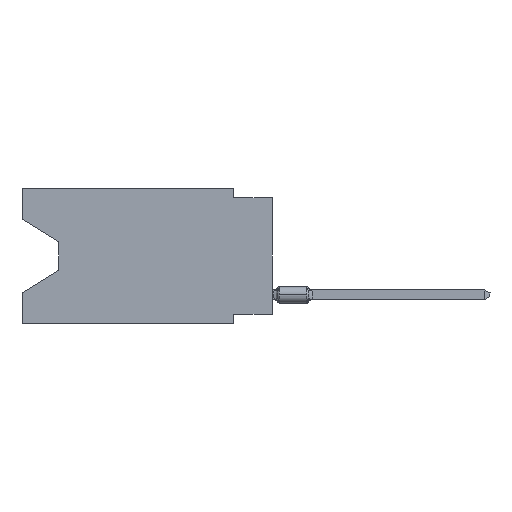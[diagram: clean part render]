
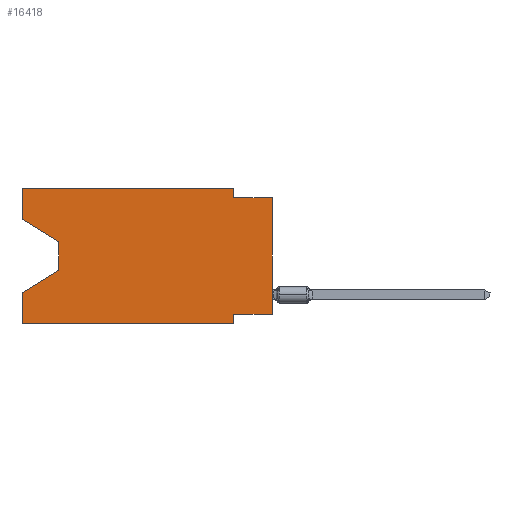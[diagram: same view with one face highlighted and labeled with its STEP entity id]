
A CAD part, left-side view. The second image highlights one B-rep face of the part: STEP entity #16418.
In plain terms, the highlighted planar face has unit normal (-1, 0, 0).
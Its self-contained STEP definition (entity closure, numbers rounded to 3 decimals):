
#2 = LINE ( 'NONE', #21927, #46086 ) ;
#419 = ORIENTED_EDGE ( 'NONE', *, *, #3825, .F. ) ;
#1229 = VERTEX_POINT ( 'NONE', #23318 ) ;
#1656 = EDGE_CURVE ( 'NONE', #2385, #42444, #24972, .T. ) ;
#2029 = DIRECTION ( 'NONE',  ( 0., -1., 0. ) ) ;
#2385 = VERTEX_POINT ( 'NONE', #20226 ) ;
#3034 = CARTESIAN_POINT ( 'NONE',  ( 0., 2.54, -0.635 ) ) ;
#3571 = FACE_OUTER_BOUND ( 'NONE', #19895, .T. ) ;
#3825 = EDGE_CURVE ( 'NONE', #16563, #17031, #41467, .T. ) ;
#4447 = CARTESIAN_POINT ( 'NONE',  ( 0., 16.383, -8.89 ) ) ;
#4960 = EDGE_CURVE ( 'NONE', #27986, #5207, #32942, .T. ) ;
#5034 = DIRECTION ( 'NONE',  ( 0., 0., -1. ) ) ;
#5039 = ORIENTED_EDGE ( 'NONE', *, *, #4960, .T. ) ;
#5207 = VERTEX_POINT ( 'NONE', #31903 ) ;
#5421 = EDGE_CURVE ( 'NONE', #34486, #16563, #33368, .T. ) ;
#6289 = CARTESIAN_POINT ( 'NONE',  ( 0., 2.54, 0. ) ) ;
#6742 = ORIENTED_EDGE ( 'NONE', *, *, #1656, .T. ) ;
#8079 = ORIENTED_EDGE ( 'NONE', *, *, #27293, .F. ) ;
#8285 = AXIS2_PLACEMENT_3D ( 'NONE', #18919, #30460, #45799 ) ;
#8574 = ORIENTED_EDGE ( 'NONE', *, *, #30937, .F. ) ;
#9012 = LINE ( 'NONE', #24568, #41256 ) ;
#9059 = VECTOR ( 'NONE', #11866, 1000. ) ;
#9601 = LINE ( 'NONE', #48049, #35440 ) ;
#9666 = DIRECTION ( 'NONE',  ( 0., -0.855, -0.519 ) ) ;
#10610 = DIRECTION ( 'NONE',  ( 0., 0., 1. ) ) ;
#10812 = DIRECTION ( 'NONE',  ( 0., 0., -1. ) ) ;
#11359 = LINE ( 'NONE', #34215, #9059 ) ;
#11866 = DIRECTION ( 'NONE',  ( 0., -1., 0. ) ) ;
#13371 = DIRECTION ( 'NONE',  ( 0., 0., 1. ) ) ;
#13841 = DIRECTION ( 'NONE',  ( 0., 0.855, -0.519 ) ) ;
#14010 = VECTOR ( 'NONE', #18046, 1000. ) ;
#14646 = VECTOR ( 'NONE', #5034, 1000. ) ;
#16297 = ORIENTED_EDGE ( 'NONE', *, *, #33588, .T. ) ;
#16418 = ADVANCED_FACE ( 'NONE', ( #3571 ), #38516, .F. ) ;
#16563 = VERTEX_POINT ( 'NONE', #47769 ) ;
#16640 = LINE ( 'NONE', #20636, #32888 ) ;
#16718 = CARTESIAN_POINT ( 'NONE',  ( 0., 0., -8.255 ) ) ;
#16900 = ORIENTED_EDGE ( 'NONE', *, *, #31813, .F. ) ;
#17031 = VERTEX_POINT ( 'NONE', #22737 ) ;
#17800 = CARTESIAN_POINT ( 'NONE',  ( 0., 13.97, -3.505 ) ) ;
#18046 = DIRECTION ( 'NONE',  ( 0., 0., -1. ) ) ;
#18372 = CARTESIAN_POINT ( 'NONE',  ( 0., 2.54, -8.89 ) ) ;
#18919 = CARTESIAN_POINT ( 'NONE',  ( 0., 16.383, 0. ) ) ;
#19345 = ORIENTED_EDGE ( 'NONE', *, *, #33767, .T. ) ;
#19820 = VERTEX_POINT ( 'NONE', #6289 ) ;
#19895 = EDGE_LOOP ( 'NONE', ( #6742, #19345, #5039, #42087, #16297, #419, #42692, #38573, #16900, #28901, #8079, #8574 ) ) ;
#20226 = CARTESIAN_POINT ( 'NONE',  ( 0., 16.383, -2.038 ) ) ;
#20636 = CARTESIAN_POINT ( 'NONE',  ( 0., 16.383, 0. ) ) ;
#21433 = VECTOR ( 'NONE', #26128, 1000. ) ;
#21927 = CARTESIAN_POINT ( 'NONE',  ( 0., 0., 0. ) ) ;
#22737 = CARTESIAN_POINT ( 'NONE',  ( 0., 2.54, -8.89 ) ) ;
#23318 = CARTESIAN_POINT ( 'NONE',  ( 0., 16.383, 0. ) ) ;
#24405 = CARTESIAN_POINT ( 'NONE',  ( 0., 0., -0.635 ) ) ;
#24568 = CARTESIAN_POINT ( 'NONE',  ( 0., 16.383, -8.89 ) ) ;
#24972 = LINE ( 'NONE', #28251, #33145 ) ;
#25901 = EDGE_CURVE ( 'NONE', #27479, #5207, #37201, .T. ) ;
#26128 = DIRECTION ( 'NONE',  ( 0., 0., 1. ) ) ;
#26996 = CARTESIAN_POINT ( 'NONE',  ( 0., 13.97, -5.385 ) ) ;
#27293 = EDGE_CURVE ( 'NONE', #1229, #19820, #16640, .T. ) ;
#27479 = VERTEX_POINT ( 'NONE', #4447 ) ;
#27986 = VERTEX_POINT ( 'NONE', #26996 ) ;
#28251 = CARTESIAN_POINT ( 'NONE',  ( 0., 16.383, -2.038 ) ) ;
#28901 = ORIENTED_EDGE ( 'NONE', *, *, #32006, .F. ) ;
#29904 = CARTESIAN_POINT ( 'NONE',  ( 0., 16.383, 0. ) ) ;
#30289 = VECTOR ( 'NONE', #32386, 1000. ) ;
#30460 = DIRECTION ( 'NONE',  ( 1., 0., 0. ) ) ;
#30937 = EDGE_CURVE ( 'NONE', #2385, #1229, #9601, .T. ) ;
#31813 = EDGE_CURVE ( 'NONE', #40453, #38855, #11359, .T. ) ;
#31903 = CARTESIAN_POINT ( 'NONE',  ( 0., 16.383, -6.852 ) ) ;
#32006 = EDGE_CURVE ( 'NONE', #19820, #40453, #43993, .T. ) ;
#32386 = DIRECTION ( 'NONE',  ( 0., 1., 0. ) ) ;
#32888 = VECTOR ( 'NONE', #2029, 1000. ) ;
#32942 = LINE ( 'NONE', #48265, #49487 ) ;
#33145 = VECTOR ( 'NONE', #9666, 1000. ) ;
#33368 = LINE ( 'NONE', #48706, #30289 ) ;
#33432 = EDGE_CURVE ( 'NONE', #34486, #38855, #2, .T. ) ;
#33588 = EDGE_CURVE ( 'NONE', #27479, #17031, #9012, .T. ) ;
#33767 = EDGE_CURVE ( 'NONE', #42444, #27986, #48945, .T. ) ;
#34215 = CARTESIAN_POINT ( 'NONE',  ( 0., 0., -0.635 ) ) ;
#34486 = VERTEX_POINT ( 'NONE', #16718 ) ;
#35440 = VECTOR ( 'NONE', #13371, 1000. ) ;
#36620 = VECTOR ( 'NONE', #10812, 1000. ) ;
#37201 = LINE ( 'NONE', #29904, #21433 ) ;
#38516 = PLANE ( 'NONE',  #8285 ) ;
#38573 = ORIENTED_EDGE ( 'NONE', *, *, #33432, .T. ) ;
#38855 = VERTEX_POINT ( 'NONE', #24405 ) ;
#39479 = CARTESIAN_POINT ( 'NONE',  ( 0., 2.54, 0. ) ) ;
#40168 = DIRECTION ( 'NONE',  ( 0., -1., 0. ) ) ;
#40453 = VERTEX_POINT ( 'NONE', #3034 ) ;
#40880 = CARTESIAN_POINT ( 'NONE',  ( 0., 13.97, -3.505 ) ) ;
#41256 = VECTOR ( 'NONE', #40168, 1000. ) ;
#41467 = LINE ( 'NONE', #18372, #36620 ) ;
#42087 = ORIENTED_EDGE ( 'NONE', *, *, #25901, .F. ) ;
#42444 = VERTEX_POINT ( 'NONE', #40880 ) ;
#42692 = ORIENTED_EDGE ( 'NONE', *, *, #5421, .F. ) ;
#43993 = LINE ( 'NONE', #39479, #14646 ) ;
#45799 = DIRECTION ( 'NONE',  ( 0., 0., -1. ) ) ;
#46086 = VECTOR ( 'NONE', #10610, 1000. ) ;
#47769 = CARTESIAN_POINT ( 'NONE',  ( 0., 2.54, -8.255 ) ) ;
#48049 = CARTESIAN_POINT ( 'NONE',  ( 0., 16.383, 0. ) ) ;
#48265 = CARTESIAN_POINT ( 'NONE',  ( 0., 13.97, -5.385 ) ) ;
#48706 = CARTESIAN_POINT ( 'NONE',  ( 0., 0., -8.255 ) ) ;
#48945 = LINE ( 'NONE', #17800, #14010 ) ;
#49487 = VECTOR ( 'NONE', #13841, 1000. ) ;
